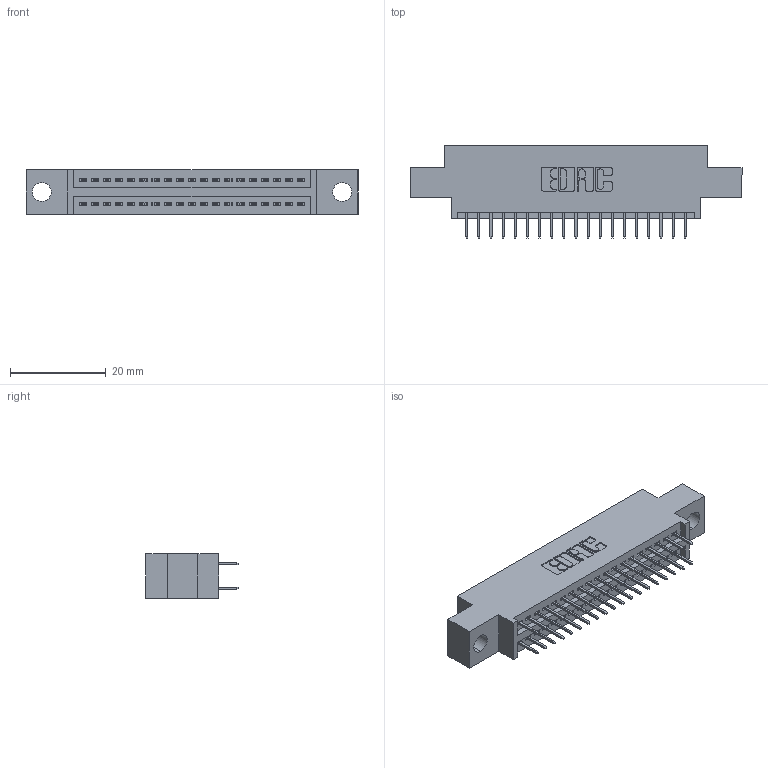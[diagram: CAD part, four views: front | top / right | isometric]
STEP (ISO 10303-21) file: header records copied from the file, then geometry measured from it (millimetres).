
FILE_DESCRIPTION (( 'STEP AP203' ), '1' );
FILE_NAME ('345-038-524-804.STEP', '2021-05-20T00:45:36', ( '' ), ( '' ), 'SwSTEP 2.0', 'SolidWorks 2020', '' );
FILE_SCHEMA (( 'CONFIG_CONTROL_DESIGN' ));
Length unit declared in the file: inch
Products named in the file (3): 345 Part_0.170 Offset - 0.156 Dia-TI; 345-038-524-804; 345-292-001_345-293-124
Assembly tree (39 placements, depth 2):
  345-038-524-804
    345 Part_0.170 Offset - 0.156 Dia-TI
    345-292-001_345-293-124  x38
Bounding box: 69.47 x 19.35 x 9.4 mm (x, y, z)
Volume: 6258 mm3; surface area: 8648.1 mm2
Topology: 39 solids, 39 shells, 2196 faces, 6203 edges, 3982 vertices
Faces by surface type: plane 1580, cylinder 616
Entity records: 18629 total; most frequent: CARTESIAN_POINT 3150, ORIENTED_EDGE 3082, DIRECTION 2805, EDGE_CURVE 1541, LINE 1337, VECTOR 1337, VERTEX_POINT 1022, AXIS2_PLACEMENT_3D 734
